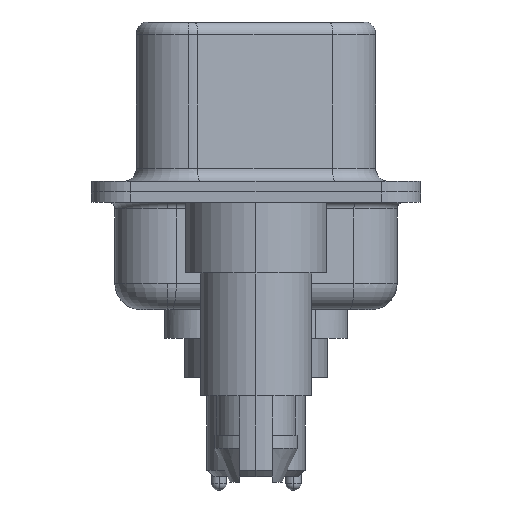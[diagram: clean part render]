
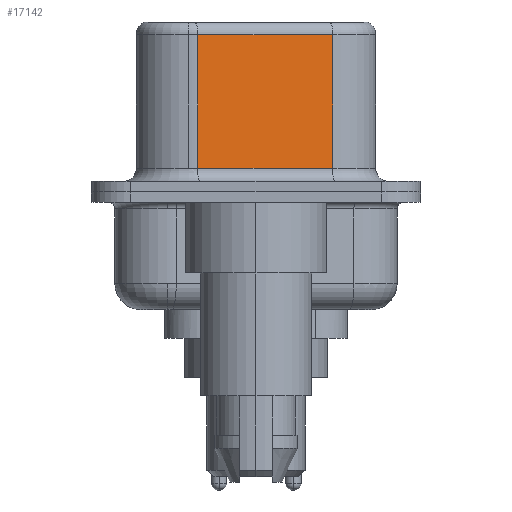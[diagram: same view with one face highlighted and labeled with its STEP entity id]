
A CAD part, left-side view. The second image highlights one B-rep face of the part: STEP entity #17142.
In plain terms, the highlighted planar face has unit normal (-0.985, -0.174, 0).
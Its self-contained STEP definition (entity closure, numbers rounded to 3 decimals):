
#492 = DIRECTION ( 'NONE',  ( 0.174, -0.985, 0. ) ) ;
#1878 = EDGE_LOOP ( 'NONE', ( #13787, #15214, #20610, #8985 ) ) ;
#1911 = LINE ( 'NONE', #12510, #19679 ) ;
#2263 = LINE ( 'NONE', #5449, #19998 ) ;
#3118 = AXIS2_PLACEMENT_3D ( 'NONE', #3204, #22086, #12018 ) ;
#3204 = CARTESIAN_POINT ( 'NONE',  ( 4.585, -2.927, 6.52 ) ) ;
#3685 = DIRECTION ( 'NONE',  ( -0.174, 0.985, 0. ) ) ;
#4811 = DIRECTION ( 'NONE',  ( 0., 0., -1. ) ) ;
#4920 = VERTEX_POINT ( 'NONE', #14315 ) ;
#4941 = CARTESIAN_POINT ( 'NONE',  ( 4.585, -2.927, 6.02 ) ) ;
#5022 = PLANE ( 'NONE',  #3118 ) ;
#5449 = CARTESIAN_POINT ( 'NONE',  ( 4.585, -2.927, 6.02 ) ) ;
#5889 = VERTEX_POINT ( 'NONE', #16809 ) ;
#5980 = EDGE_CURVE ( 'NONE', #5889, #4920, #19538, .T. ) ;
#7620 = EDGE_CURVE ( 'NONE', #19635, #5889, #2263, .T. ) ;
#8985 = ORIENTED_EDGE ( 'NONE', *, *, #16006, .T. ) ;
#9105 = DIRECTION ( 'NONE',  ( 0., 0., -1. ) ) ;
#10060 = VECTOR ( 'NONE', #492, 1000. ) ;
#10276 = CARTESIAN_POINT ( 'NONE',  ( 4.585, -2.927, 0.9 ) ) ;
#10641 = LINE ( 'NONE', #21071, #10060 ) ;
#12018 = DIRECTION ( 'NONE',  ( -0.174, 0.985, 0. ) ) ;
#12510 = CARTESIAN_POINT ( 'NONE',  ( 4.585, -2.927, 6.52 ) ) ;
#13435 = CARTESIAN_POINT ( 'NONE',  ( 3.675, 2.233, 6.52 ) ) ;
#13787 = ORIENTED_EDGE ( 'NONE', *, *, #15978, .F. ) ;
#13804 = FACE_OUTER_BOUND ( 'NONE', #1878, .T. ) ;
#14315 = CARTESIAN_POINT ( 'NONE',  ( 3.675, 2.233, 0.9 ) ) ;
#15214 = ORIENTED_EDGE ( 'NONE', *, *, #7620, .T. ) ;
#15978 = EDGE_CURVE ( 'NONE', #19635, #18674, #1911, .T. ) ;
#16006 = EDGE_CURVE ( 'NONE', #4920, #18674, #10641, .T. ) ;
#16137 = VECTOR ( 'NONE', #4811, 1000. ) ;
#16809 = CARTESIAN_POINT ( 'NONE',  ( 3.675, 2.233, 6.02 ) ) ;
#17142 = ADVANCED_FACE ( 'NONE', ( #13804 ), #5022, .F. ) ;
#18674 = VERTEX_POINT ( 'NONE', #10276 ) ;
#19538 = LINE ( 'NONE', #13435, #16137 ) ;
#19635 = VERTEX_POINT ( 'NONE', #4941 ) ;
#19679 = VECTOR ( 'NONE', #9105, 1000. ) ;
#19998 = VECTOR ( 'NONE', #3685, 1000. ) ;
#20610 = ORIENTED_EDGE ( 'NONE', *, *, #5980, .T. ) ;
#21071 = CARTESIAN_POINT ( 'NONE',  ( 4.585, -2.927, 0.9 ) ) ;
#22086 = DIRECTION ( 'NONE',  ( 0.985, 0.174, 0. ) ) ;
